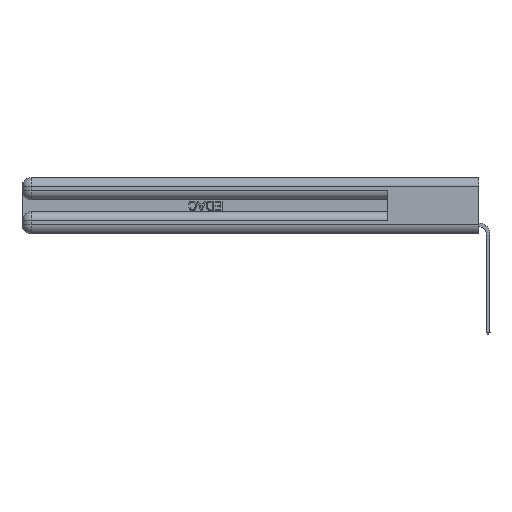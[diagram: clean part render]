
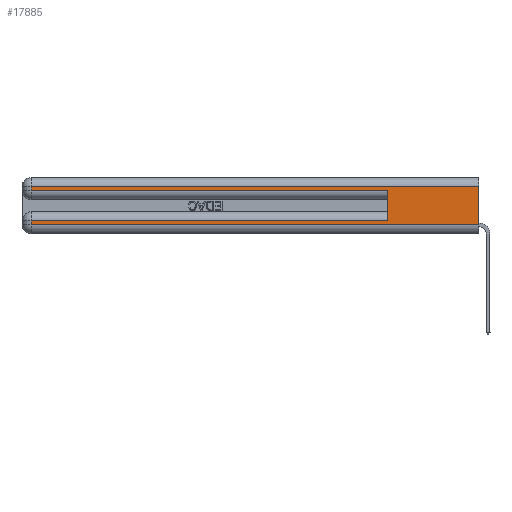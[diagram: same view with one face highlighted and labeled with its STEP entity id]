
A CAD part, left-side view. The second image highlights one B-rep face of the part: STEP entity #17885.
In plain terms, the highlighted planar face has unit normal (-1, 0, 0).
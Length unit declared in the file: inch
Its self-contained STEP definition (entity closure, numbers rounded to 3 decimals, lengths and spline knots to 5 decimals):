
#197 = ORIENTED_EDGE ( 'NONE', *, *, #26123, .T. ) ;
#199 = VECTOR ( 'NONE', #28841, 39.37008 ) ;
#921 = PLANE ( 'NONE',  #8452 ) ;
#930 = EDGE_CURVE ( 'NONE', #15861, #28344, #27299, .T. ) ;
#1372 = LINE ( 'NONE', #30354, #6968 ) ;
#1816 = EDGE_CURVE ( 'NONE', #9978, #28344, #1372, .T. ) ;
#2550 = EDGE_CURVE ( 'NONE', #10169, #25706, #28958, .T. ) ;
#3323 = CARTESIAN_POINT ( 'NONE',  ( 0., 0.6, 0.085 ) ) ;
#3711 = EDGE_CURVE ( 'NONE', #15861, #10169, #7155, .T. ) ;
#3713 = LINE ( 'NONE', #8814, #16068 ) ;
#4376 = VECTOR ( 'NONE', #24378, 39.37008 ) ;
#4924 = DIRECTION ( 'NONE',  ( 0., 1., 0. ) ) ;
#5584 = DIRECTION ( 'NONE',  ( 0., 0., 1. ) ) ;
#5641 = EDGE_CURVE ( 'NONE', #9349, #19187, #16991, .T. ) ;
#5662 = CARTESIAN_POINT ( 'NONE',  ( 0., 0., 0.37 ) ) ;
#6968 = VECTOR ( 'NONE', #11552, 39.37008 ) ;
#7155 = LINE ( 'NONE', #26495, #25903 ) ;
#7424 = ORIENTED_EDGE ( 'NONE', *, *, #18530, .T. ) ;
#7764 = CARTESIAN_POINT ( 'NONE',  ( 0., 0., 0.31 ) ) ;
#8452 = AXIS2_PLACEMENT_3D ( 'NONE', #5662, #17404, #29739 ) ;
#8814 = CARTESIAN_POINT ( 'NONE',  ( 0., 2.94, 0.37 ) ) ;
#9349 = VERTEX_POINT ( 'NONE', #11494 ) ;
#9545 = LINE ( 'NONE', #7764, #199 ) ;
#9978 = VERTEX_POINT ( 'NONE', #14865 ) ;
#10169 = VERTEX_POINT ( 'NONE', #18310 ) ;
#10290 = FACE_OUTER_BOUND ( 'NONE', #30200, .T. ) ;
#10688 = ORIENTED_EDGE ( 'NONE', *, *, #27781, .T. ) ;
#10830 = CARTESIAN_POINT ( 'NONE',  ( 0., 0.6, 0.145 ) ) ;
#11057 = CARTESIAN_POINT ( 'NONE',  ( 0., 2.94, 0.31 ) ) ;
#11494 = CARTESIAN_POINT ( 'NONE',  ( 0., 0., 0.31 ) ) ;
#11552 = DIRECTION ( 'NONE',  ( 0., -1., 0. ) ) ;
#13095 = DIRECTION ( 'NONE',  ( 0., 0., -1. ) ) ;
#13187 = LINE ( 'NONE', #15247, #28453 ) ;
#14099 = ORIENTED_EDGE ( 'NONE', *, *, #5641, .F. ) ;
#14677 = CARTESIAN_POINT ( 'NONE',  ( 0., 2.94, 0.06 ) ) ;
#14865 = CARTESIAN_POINT ( 'NONE',  ( 0., 2.94, 0.285 ) ) ;
#15247 = CARTESIAN_POINT ( 'NONE',  ( 0., 0., 0.06 ) ) ;
#15861 = VERTEX_POINT ( 'NONE', #3323 ) ;
#16068 = VECTOR ( 'NONE', #13095, 39.37008 ) ;
#16180 = ORIENTED_EDGE ( 'NONE', *, *, #1816, .T. ) ;
#16991 = LINE ( 'NONE', #17154, #20227 ) ;
#17154 = CARTESIAN_POINT ( 'NONE',  ( 0., 0., 0.37 ) ) ;
#17404 = DIRECTION ( 'NONE',  ( 1., 0., 0. ) ) ;
#17885 = ADVANCED_FACE ( 'NONE', ( #10290 ), #921, .F. ) ;
#18310 = CARTESIAN_POINT ( 'NONE',  ( 0., 2.94, 0.085 ) ) ;
#18530 = EDGE_CURVE ( 'NONE', #29655, #9978, #3713, .T. ) ;
#18703 = ORIENTED_EDGE ( 'NONE', *, *, #3711, .T. ) ;
#19187 = VERTEX_POINT ( 'NONE', #27534 ) ;
#19989 = DIRECTION ( 'NONE',  ( 0., -1., 0. ) ) ;
#20227 = VECTOR ( 'NONE', #26504, 39.37008 ) ;
#21049 = VECTOR ( 'NONE', #5584, 39.37008 ) ;
#24378 = DIRECTION ( 'NONE',  ( 0., 0., -1. ) ) ;
#25706 = VERTEX_POINT ( 'NONE', #14677 ) ;
#25903 = VECTOR ( 'NONE', #4924, 39.37008 ) ;
#26123 = EDGE_CURVE ( 'NONE', #25706, #19187, #13187, .T. ) ;
#26495 = CARTESIAN_POINT ( 'NONE',  ( 0., 0., 0.085 ) ) ;
#26504 = DIRECTION ( 'NONE',  ( 0., 0., -1. ) ) ;
#27299 = LINE ( 'NONE', #10830, #21049 ) ;
#27348 = ORIENTED_EDGE ( 'NONE', *, *, #2550, .T. ) ;
#27534 = CARTESIAN_POINT ( 'NONE',  ( 0., 0., 0.06 ) ) ;
#27781 = EDGE_CURVE ( 'NONE', #9349, #29655, #9545, .T. ) ;
#28344 = VERTEX_POINT ( 'NONE', #29877 ) ;
#28453 = VECTOR ( 'NONE', #19989, 39.37008 ) ;
#28841 = DIRECTION ( 'NONE',  ( 0., 1., 0. ) ) ;
#28958 = LINE ( 'NONE', #29277, #4376 ) ;
#29277 = CARTESIAN_POINT ( 'NONE',  ( 0., 2.94, 0.37 ) ) ;
#29655 = VERTEX_POINT ( 'NONE', #11057 ) ;
#29739 = DIRECTION ( 'NONE',  ( 0., 0., -1. ) ) ;
#29877 = CARTESIAN_POINT ( 'NONE',  ( 0., 0.6, 0.285 ) ) ;
#30200 = EDGE_LOOP ( 'NONE', ( #14099, #10688, #7424, #16180, #30480, #18703, #27348, #197 ) ) ;
#30354 = CARTESIAN_POINT ( 'NONE',  ( 0., 0., 0.285 ) ) ;
#30480 = ORIENTED_EDGE ( 'NONE', *, *, #930, .F. ) ;
